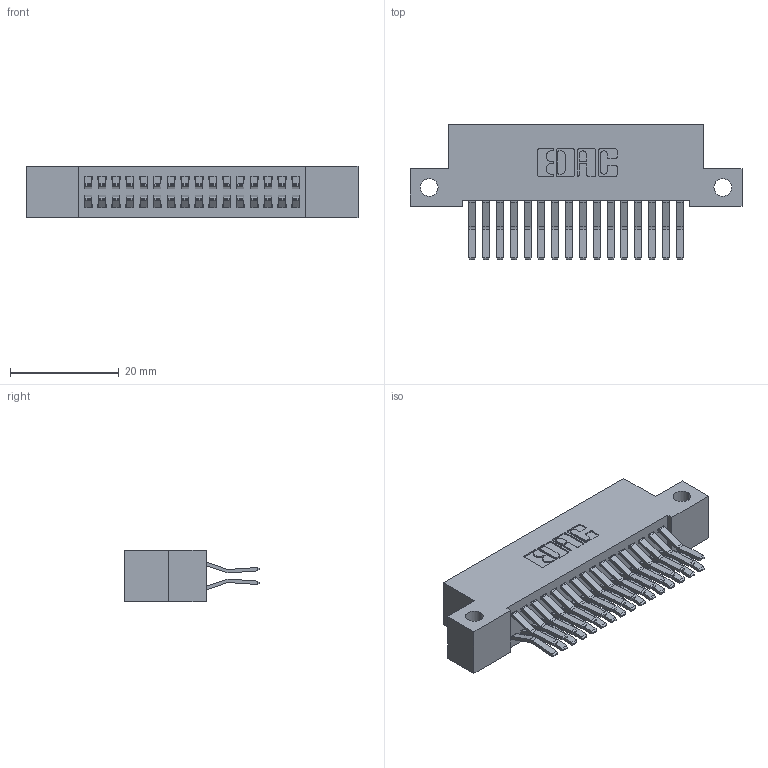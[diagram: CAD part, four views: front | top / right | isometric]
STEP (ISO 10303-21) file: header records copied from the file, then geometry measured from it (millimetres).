
FILE_DESCRIPTION (( 'STEP AP203' ), '1' );
FILE_NAME ('342-032-560-212.STEP', '2018-08-11T17:31:19', ( '' ), ( '' ), 'SwSTEP 2.0', 'SolidWorks 2016', '' );
FILE_SCHEMA (( 'CONFIG_CONTROL_DESIGN' ));
Length unit declared in the file: inch
Products named in the file (3): 342 Part_Side Mount; 345-292-001_560 Tail; 342-032-560-212
Assembly tree (33 placements, depth 2):
  342-032-560-212
    342 Part_Side Mount
    345-292-001_560 Tail  x32
Bounding box: 60.96 x 24.78 x 9.4 mm (x, y, z)
Volume: 5490.3 mm3; surface area: 8640.2 mm2
Topology: 33 solids, 33 shells, 1838 faces, 5451 edges, 3590 vertices
Faces by surface type: plane 1218, cylinder 620
Entity records: 13615 total; most frequent: CARTESIAN_POINT 2286, ORIENTED_EDGE 2222, DIRECTION 2003, EDGE_CURVE 1111, VECTOR 979, LINE 979, VERTEX_POINT 738, AXIS2_PLACEMENT_3D 512
